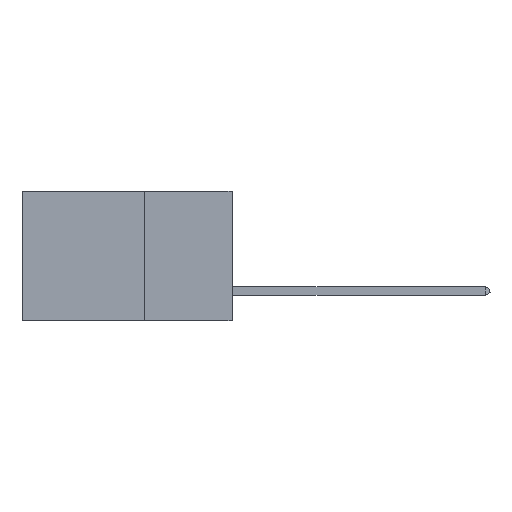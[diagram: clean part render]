
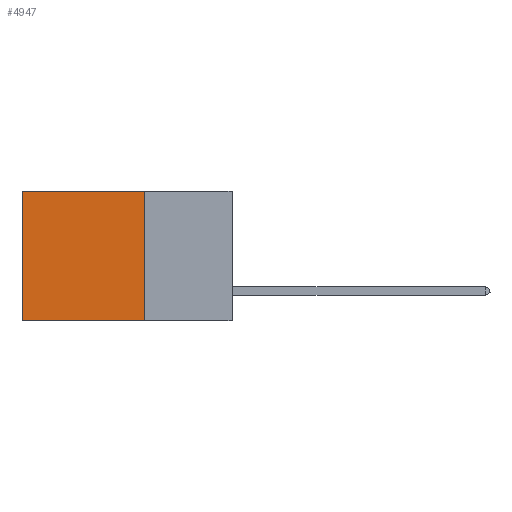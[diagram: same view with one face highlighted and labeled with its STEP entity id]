
A CAD part, left-side view. The second image highlights one B-rep face of the part: STEP entity #4947.
In plain terms, the highlighted planar face has unit normal (-1, 0, 0).
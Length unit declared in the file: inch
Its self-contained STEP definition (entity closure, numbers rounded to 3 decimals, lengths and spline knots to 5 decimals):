
#9 = DIRECTION ( 'NONE',  ( 0., 0., -1. ) ) ;
#656 = EDGE_CURVE ( 'NONE', #4322, #2431, #10811, .T. ) ;
#672 = ORIENTED_EDGE ( 'NONE', *, *, #2437, .T. ) ;
#1138 = VECTOR ( 'NONE', #9, 39.37008 ) ;
#1628 = VECTOR ( 'NONE', #3294, 39.37008 ) ;
#2217 = CARTESIAN_POINT ( 'NONE',  ( 0.2875, 0.25, -0.37 ) ) ;
#2431 = VERTEX_POINT ( 'NONE', #6447 ) ;
#2437 = EDGE_CURVE ( 'NONE', #6061, #4322, #13687, .T. ) ;
#2782 = CARTESIAN_POINT ( 'NONE',  ( 0.2875, 0.25, 0. ) ) ;
#3294 = DIRECTION ( 'NONE',  ( 0., 1., 0. ) ) ;
#3305 = DIRECTION ( 'NONE',  ( 1., 0., 0. ) ) ;
#3551 = CARTESIAN_POINT ( 'NONE',  ( 0.2875, 0.6, 0. ) ) ;
#4188 = LINE ( 'NONE', #4560, #1138 ) ;
#4286 = DIRECTION ( 'NONE',  ( 0., 1., 0. ) ) ;
#4322 = VERTEX_POINT ( 'NONE', #11911 ) ;
#4416 = PLANE ( 'NONE',  #6056 ) ;
#4560 = CARTESIAN_POINT ( 'NONE',  ( 0.2875, 0.25, 0. ) ) ;
#4725 = DIRECTION ( 'NONE',  ( 0., 0., -1. ) ) ;
#4947 = ADVANCED_FACE ( 'NONE', ( #5698 ), #4416, .F. ) ;
#5698 = FACE_OUTER_BOUND ( 'NONE', #7615, .T. ) ;
#5714 = CARTESIAN_POINT ( 'NONE',  ( 0.2875, 0.25, 0. ) ) ;
#6056 = AXIS2_PLACEMENT_3D ( 'NONE', #12441, #3305, #11214 ) ;
#6061 = VERTEX_POINT ( 'NONE', #2782 ) ;
#6447 = CARTESIAN_POINT ( 'NONE',  ( 0.2875, 0.6, -0.37 ) ) ;
#7342 = ORIENTED_EDGE ( 'NONE', *, *, #656, .T. ) ;
#7564 = VERTEX_POINT ( 'NONE', #2217 ) ;
#7615 = EDGE_LOOP ( 'NONE', ( #7342, #14109, #13825, #672 ) ) ;
#9860 = VECTOR ( 'NONE', #4286, 39.37008 ) ;
#10811 = LINE ( 'NONE', #3551, #12463 ) ;
#11214 = DIRECTION ( 'NONE',  ( 0., 0., -1. ) ) ;
#11229 = EDGE_CURVE ( 'NONE', #7564, #2431, #13304, .T. ) ;
#11911 = CARTESIAN_POINT ( 'NONE',  ( 0.2875, 0.6, 0. ) ) ;
#12441 = CARTESIAN_POINT ( 'NONE',  ( 0.2875, 0.25, 0. ) ) ;
#12463 = VECTOR ( 'NONE', #4725, 39.37008 ) ;
#13304 = LINE ( 'NONE', #13644, #9860 ) ;
#13644 = CARTESIAN_POINT ( 'NONE',  ( 0.2875, 0.25, -0.37 ) ) ;
#13687 = LINE ( 'NONE', #5714, #1628 ) ;
#13825 = ORIENTED_EDGE ( 'NONE', *, *, #13920, .F. ) ;
#13920 = EDGE_CURVE ( 'NONE', #6061, #7564, #4188, .T. ) ;
#14109 = ORIENTED_EDGE ( 'NONE', *, *, #11229, .F. ) ;
